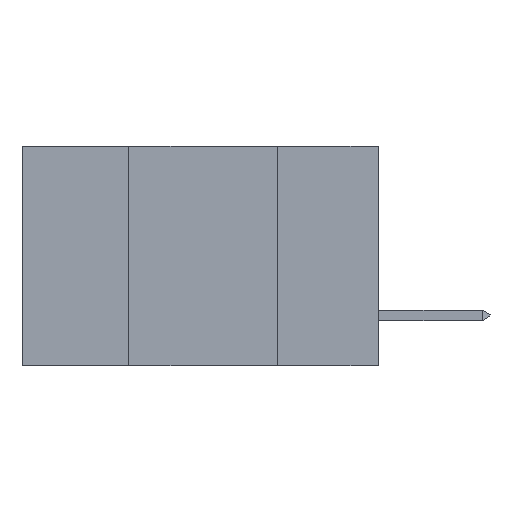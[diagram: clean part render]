
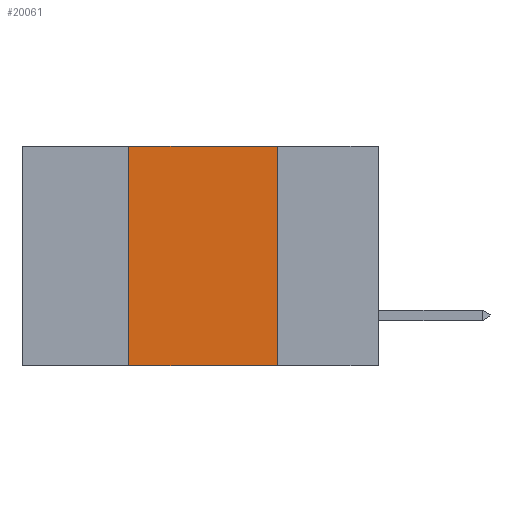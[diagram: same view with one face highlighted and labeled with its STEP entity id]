
A CAD part, left-side view. The second image highlights one B-rep face of the part: STEP entity #20061.
In plain terms, the highlighted planar face has unit normal (-1, 0, 0).
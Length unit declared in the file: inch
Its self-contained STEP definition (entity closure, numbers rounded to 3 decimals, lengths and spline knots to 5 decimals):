
#195 = DIRECTION ( 'NONE',  ( 0., -1., 0. ) ) ;
#254 = CARTESIAN_POINT ( 'NONE',  ( 0., 0.17, -0.37 ) ) ;
#2701 = ORIENTED_EDGE ( 'NONE', *, *, #7250, .F. ) ;
#4617 = EDGE_CURVE ( 'NONE', #13107, #19186, #5606, .T. ) ;
#5323 = CARTESIAN_POINT ( 'NONE',  ( 0., 0.17, -0.37 ) ) ;
#5606 = LINE ( 'NONE', #14854, #7675 ) ;
#6046 = ORIENTED_EDGE ( 'NONE', *, *, #12814, .F. ) ;
#6304 = VECTOR ( 'NONE', #19762, 39.37008 ) ;
#6367 = ORIENTED_EDGE ( 'NONE', *, *, #10381, .F. ) ;
#7250 = EDGE_CURVE ( 'NONE', #14820, #19186, #13141, .T. ) ;
#7675 = VECTOR ( 'NONE', #195, 39.37008 ) ;
#8480 = ORIENTED_EDGE ( 'NONE', *, *, #4617, .T. ) ;
#9022 = EDGE_LOOP ( 'NONE', ( #2701, #6046, #6367, #8480 ) ) ;
#10150 = DIRECTION ( 'NONE',  ( 0., 0., -1. ) ) ;
#10381 = EDGE_CURVE ( 'NONE', #13107, #13395, #17682, .T. ) ;
#11614 = LINE ( 'NONE', #14841, #6304 ) ;
#11633 = DIRECTION ( 'NONE',  ( 1., 0., 0. ) ) ;
#12639 = DIRECTION ( 'NONE',  ( 0., 0., 1. ) ) ;
#12814 = EDGE_CURVE ( 'NONE', #13395, #14820, #11614, .T. ) ;
#13107 = VERTEX_POINT ( 'NONE', #14786 ) ;
#13141 = LINE ( 'NONE', #5323, #16866 ) ;
#13395 = VERTEX_POINT ( 'NONE', #14134 ) ;
#13556 = CARTESIAN_POINT ( 'NONE',  ( 0., 0.6, 0. ) ) ;
#13658 = AXIS2_PLACEMENT_3D ( 'NONE', #13556, #11633, #16878 ) ;
#14100 = CARTESIAN_POINT ( 'NONE',  ( 0., 0.17, 0. ) ) ;
#14134 = CARTESIAN_POINT ( 'NONE',  ( 0., 0.42, 0. ) ) ;
#14786 = CARTESIAN_POINT ( 'NONE',  ( 0., 0.42, -0.37 ) ) ;
#14820 = VERTEX_POINT ( 'NONE', #14100 ) ;
#14841 = CARTESIAN_POINT ( 'NONE',  ( 0., 0.6, 0. ) ) ;
#14854 = CARTESIAN_POINT ( 'NONE',  ( 0., 0.6, -0.37 ) ) ;
#16866 = VECTOR ( 'NONE', #10150, 39.37008 ) ;
#16878 = DIRECTION ( 'NONE',  ( 0., 0., -1. ) ) ;
#17682 = LINE ( 'NONE', #17890, #17879 ) ;
#17879 = VECTOR ( 'NONE', #12639, 39.37008 ) ;
#17890 = CARTESIAN_POINT ( 'NONE',  ( 0., 0.42, -0.37 ) ) ;
#19186 = VERTEX_POINT ( 'NONE', #254 ) ;
#19762 = DIRECTION ( 'NONE',  ( 0., -1., 0. ) ) ;
#19784 = PLANE ( 'NONE',  #13658 ) ;
#19886 = FACE_OUTER_BOUND ( 'NONE', #9022, .T. ) ;
#20061 = ADVANCED_FACE ( 'NONE', ( #19886 ), #19784, .F. ) ;
